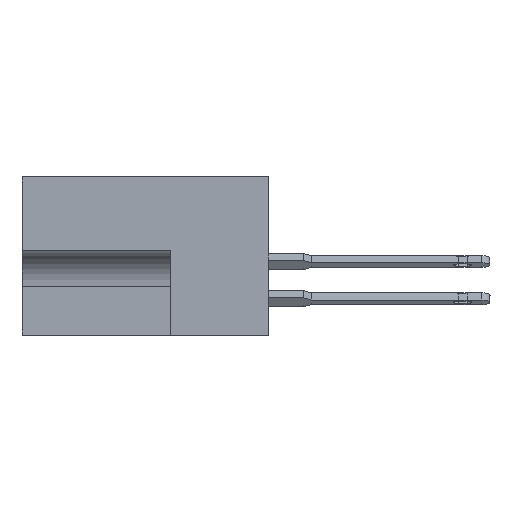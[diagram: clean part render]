
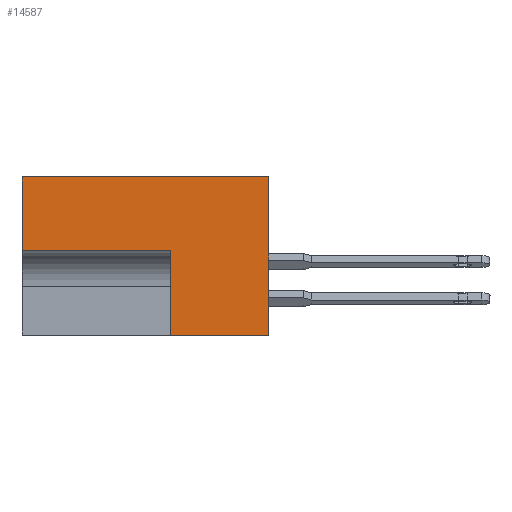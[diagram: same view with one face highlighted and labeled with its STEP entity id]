
A CAD part, left-side view. The second image highlights one B-rep face of the part: STEP entity #14587.
In plain terms, the highlighted planar face has unit normal (-1, 0, 0).
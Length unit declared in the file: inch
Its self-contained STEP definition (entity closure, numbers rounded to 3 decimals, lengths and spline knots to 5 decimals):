
#262 = CARTESIAN_POINT ( 'NONE',  ( 0., 0.453, 0. ) ) ;
#548 = EDGE_LOOP ( 'NONE', ( #12174, #19501, #15611, #26850, #18209, #7905 ) ) ;
#1671 = CARTESIAN_POINT ( 'NONE',  ( 0., 0.828, 0. ) ) ;
#1999 = EDGE_CURVE ( 'NONE', #11501, #20206, #25586, .T. ) ;
#2727 = CARTESIAN_POINT ( 'NONE',  ( 0., 0.828, 0. ) ) ;
#4155 = VECTOR ( 'NONE', #17995, 39.37008 ) ;
#4746 = AXIS2_PLACEMENT_3D ( 'NONE', #9373, #19842, #15746 ) ;
#4842 = EDGE_CURVE ( 'NONE', #5052, #10053, #17658, .T. ) ;
#5052 = VERTEX_POINT ( 'NONE', #21670 ) ;
#5358 = VECTOR ( 'NONE', #15424, 39.37008 ) ;
#5695 = EDGE_CURVE ( 'NONE', #18173, #22526, #9497, .T. ) ;
#5794 = DIRECTION ( 'NONE',  ( 0., 0., 1. ) ) ;
#6242 = VECTOR ( 'NONE', #7589, 39.37008 ) ;
#6324 = VECTOR ( 'NONE', #5794, 39.37008 ) ;
#6464 = DIRECTION ( 'NONE',  ( 0., -1., 0. ) ) ;
#7589 = DIRECTION ( 'NONE',  ( 0., 0., 1. ) ) ;
#7894 = CARTESIAN_POINT ( 'NONE',  ( 0., 0., -0.531 ) ) ;
#7905 = ORIENTED_EDGE ( 'NONE', *, *, #26578, .F. ) ;
#9373 = CARTESIAN_POINT ( 'NONE',  ( 0., 0.453, 0. ) ) ;
#9497 = LINE ( 'NONE', #13425, #6242 ) ;
#9748 = FACE_OUTER_BOUND ( 'NONE', #548, .T. ) ;
#10053 = VERTEX_POINT ( 'NONE', #15781 ) ;
#10671 = CARTESIAN_POINT ( 'NONE',  ( 0., 0.328, -0.531 ) ) ;
#11501 = VERTEX_POINT ( 'NONE', #26956 ) ;
#12174 = ORIENTED_EDGE ( 'NONE', *, *, #1999, .F. ) ;
#12629 = LINE ( 'NONE', #18179, #4155 ) ;
#13425 = CARTESIAN_POINT ( 'NONE',  ( 0., 0., 0. ) ) ;
#13646 = PLANE ( 'NONE',  #4746 ) ;
#14587 = ADVANCED_FACE ( 'NONE', ( #9748 ), #13646, .F. ) ;
#14939 = DIRECTION ( 'NONE',  ( 0., 0., 1. ) ) ;
#15424 = DIRECTION ( 'NONE',  ( 0., 1., 0. ) ) ;
#15611 = ORIENTED_EDGE ( 'NONE', *, *, #4842, .F. ) ;
#15746 = DIRECTION ( 'NONE',  ( 0., 0., -1. ) ) ;
#15781 = CARTESIAN_POINT ( 'NONE',  ( 0., 0.328, -0.248 ) ) ;
#17232 = CARTESIAN_POINT ( 'NONE',  ( 0., 0.328, -0.248 ) ) ;
#17455 = VECTOR ( 'NONE', #6464, 39.37008 ) ;
#17658 = LINE ( 'NONE', #10671, #25211 ) ;
#17995 = DIRECTION ( 'NONE',  ( 0., -1., 0. ) ) ;
#18126 = LINE ( 'NONE', #262, #17455 ) ;
#18173 = VERTEX_POINT ( 'NONE', #7894 ) ;
#18179 = CARTESIAN_POINT ( 'NONE',  ( 0., 0.453, -0.531 ) ) ;
#18209 = ORIENTED_EDGE ( 'NONE', *, *, #5695, .T. ) ;
#19501 = ORIENTED_EDGE ( 'NONE', *, *, #21930, .F. ) ;
#19777 = CARTESIAN_POINT ( 'NONE',  ( 0., 0., 0. ) ) ;
#19842 = DIRECTION ( 'NONE',  ( 1., 0., 0. ) ) ;
#20206 = VERTEX_POINT ( 'NONE', #2727 ) ;
#21670 = CARTESIAN_POINT ( 'NONE',  ( 0., 0.328, -0.531 ) ) ;
#21930 = EDGE_CURVE ( 'NONE', #10053, #11501, #25898, .T. ) ;
#22526 = VERTEX_POINT ( 'NONE', #19777 ) ;
#25211 = VECTOR ( 'NONE', #14939, 39.37008 ) ;
#25586 = LINE ( 'NONE', #1671, #6324 ) ;
#25710 = EDGE_CURVE ( 'NONE', #5052, #18173, #12629, .T. ) ;
#25898 = LINE ( 'NONE', #17232, #5358 ) ;
#26578 = EDGE_CURVE ( 'NONE', #20206, #22526, #18126, .T. ) ;
#26850 = ORIENTED_EDGE ( 'NONE', *, *, #25710, .T. ) ;
#26956 = CARTESIAN_POINT ( 'NONE',  ( 0., 0.828, -0.248 ) ) ;
